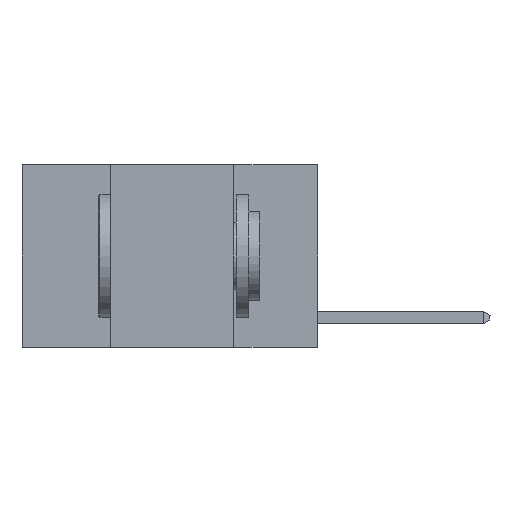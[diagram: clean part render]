
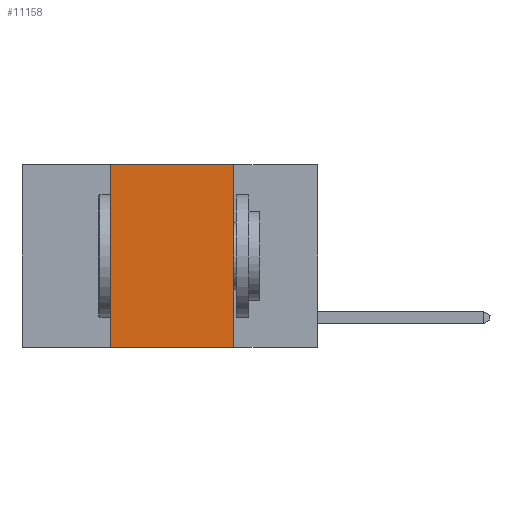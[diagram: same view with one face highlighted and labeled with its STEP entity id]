
A CAD part, left-side view. The second image highlights one B-rep face of the part: STEP entity #11158.
In plain terms, the highlighted planar face has unit normal (-1, 0, 0).
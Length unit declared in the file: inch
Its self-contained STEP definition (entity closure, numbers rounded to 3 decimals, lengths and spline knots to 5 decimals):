
#11 = AXIS2_PLACEMENT_3D ( 'NONE', #4587, #4098, #13485 ) ;
#570 = ORIENTED_EDGE ( 'NONE', *, *, #10632, .F. ) ;
#725 = CARTESIAN_POINT ( 'NONE',  ( 0., 0.17, 0. ) ) ;
#846 = VERTEX_POINT ( 'NONE', #9296 ) ;
#1349 = DIRECTION ( 'NONE',  ( 0., -1., 0. ) ) ;
#1841 = VECTOR ( 'NONE', #1349, 39.37008 ) ;
#2141 = EDGE_CURVE ( 'NONE', #846, #7553, #13761, .T. ) ;
#2718 = CARTESIAN_POINT ( 'NONE',  ( 0., 0.17, 0. ) ) ;
#3993 = VERTEX_POINT ( 'NONE', #725 ) ;
#4098 = DIRECTION ( 'NONE',  ( 1., 0., 0. ) ) ;
#4587 = CARTESIAN_POINT ( 'NONE',  ( 0., 0.6, 0. ) ) ;
#4597 = VECTOR ( 'NONE', #4938, 39.37008 ) ;
#4938 = DIRECTION ( 'NONE',  ( 0., 0., 1. ) ) ;
#5390 = ORIENTED_EDGE ( 'NONE', *, *, #6897, .T. ) ;
#5622 = LINE ( 'NONE', #12430, #1841 ) ;
#5766 = ORIENTED_EDGE ( 'NONE', *, *, #2141, .F. ) ;
#6083 = ORIENTED_EDGE ( 'NONE', *, *, #10415, .F. ) ;
#6897 = EDGE_CURVE ( 'NONE', #846, #6992, #5622, .T. ) ;
#6939 = DIRECTION ( 'NONE',  ( 0., -1., 0. ) ) ;
#6992 = VERTEX_POINT ( 'NONE', #8129 ) ;
#7013 = CARTESIAN_POINT ( 'NONE',  ( 0., 0.42, 0. ) ) ;
#7238 = DIRECTION ( 'NONE',  ( 0., 0., -1. ) ) ;
#7553 = VERTEX_POINT ( 'NONE', #10080 ) ;
#8129 = CARTESIAN_POINT ( 'NONE',  ( 0., 0.17, -0.37 ) ) ;
#8947 = FACE_OUTER_BOUND ( 'NONE', #9560, .T. ) ;
#9155 = LINE ( 'NONE', #10187, #13109 ) ;
#9296 = CARTESIAN_POINT ( 'NONE',  ( 0., 0.42, -0.37 ) ) ;
#9560 = EDGE_LOOP ( 'NONE', ( #570, #6083, #5766, #5390 ) ) ;
#10080 = CARTESIAN_POINT ( 'NONE',  ( 0., 0.42, 0. ) ) ;
#10187 = CARTESIAN_POINT ( 'NONE',  ( 0., 0.6, 0. ) ) ;
#10415 = EDGE_CURVE ( 'NONE', #7553, #3993, #9155, .T. ) ;
#10632 = EDGE_CURVE ( 'NONE', #3993, #6992, #13081, .T. ) ;
#11158 = ADVANCED_FACE ( 'NONE', ( #8947 ), #14252, .F. ) ;
#12430 = CARTESIAN_POINT ( 'NONE',  ( 0., 0.6, -0.37 ) ) ;
#12877 = VECTOR ( 'NONE', #7238, 39.37008 ) ;
#13081 = LINE ( 'NONE', #2718, #12877 ) ;
#13109 = VECTOR ( 'NONE', #6939, 39.37008 ) ;
#13485 = DIRECTION ( 'NONE',  ( 0., 0., -1. ) ) ;
#13761 = LINE ( 'NONE', #7013, #4597 ) ;
#14252 = PLANE ( 'NONE',  #11 ) ;
